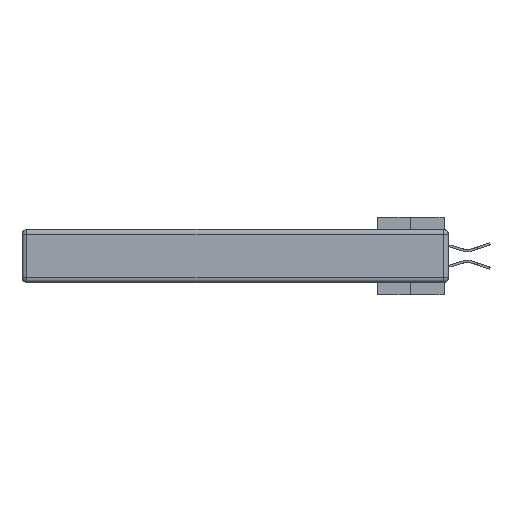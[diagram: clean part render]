
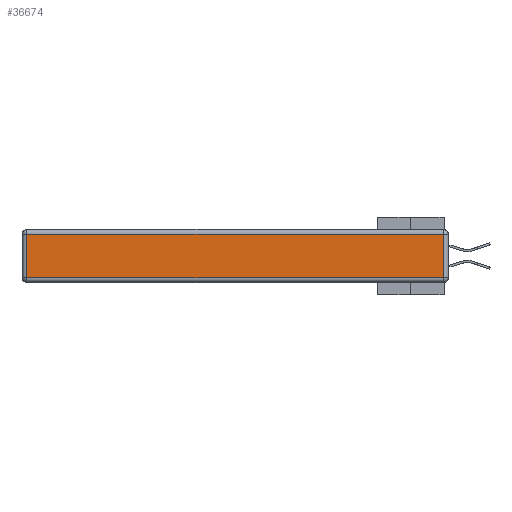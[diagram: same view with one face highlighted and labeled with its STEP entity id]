
A CAD part, left-side view. The second image highlights one B-rep face of the part: STEP entity #36674.
In plain terms, the highlighted planar face has unit normal (-1, 0, 0).
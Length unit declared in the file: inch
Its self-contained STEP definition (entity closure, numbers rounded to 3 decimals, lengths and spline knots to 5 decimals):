
#257 = CARTESIAN_POINT ( 'NONE',  ( 0., 2.72, -0.313 ) ) ;
#616 = VECTOR ( 'NONE', #44466, 39.37008 ) ;
#2462 = VERTEX_POINT ( 'NONE', #24523 ) ;
#2489 = DIRECTION ( 'NONE',  ( 0., 0., 1. ) ) ;
#2950 = CARTESIAN_POINT ( 'NONE',  ( 0., 0., -0.343 ) ) ;
#5806 = CARTESIAN_POINT ( 'NONE',  ( 0., 0.03, -0.03 ) ) ;
#5812 = DIRECTION ( 'NONE',  ( 0., 0., -1. ) ) ;
#9549 = DIRECTION ( 'NONE',  ( 0., 0., 1. ) ) ;
#11667 = AXIS2_PLACEMENT_3D ( 'NONE', #2950, #31925, #2489 ) ;
#12974 = CARTESIAN_POINT ( 'NONE',  ( 0., 2.72, -0.343 ) ) ;
#13382 = DIRECTION ( 'NONE',  ( 0., -1., 0. ) ) ;
#13912 = LINE ( 'NONE', #12974, #41670 ) ;
#15947 = CARTESIAN_POINT ( 'NONE',  ( 0., 2.75, -0.03 ) ) ;
#17008 = ORIENTED_EDGE ( 'NONE', *, *, #37620, .T. ) ;
#17960 = EDGE_LOOP ( 'NONE', ( #41388, #26431, #44806, #17008 ) ) ;
#18274 = LINE ( 'NONE', #28059, #43247 ) ;
#24523 = CARTESIAN_POINT ( 'NONE',  ( 0., 2.72, -0.03 ) ) ;
#26431 = ORIENTED_EDGE ( 'NONE', *, *, #26827, .T. ) ;
#26827 = EDGE_CURVE ( 'NONE', #36642, #41509, #18274, .T. ) ;
#28059 = CARTESIAN_POINT ( 'NONE',  ( 0., 0.03, -0.343 ) ) ;
#28369 = EDGE_CURVE ( 'NONE', #30826, #36642, #46108, .T. ) ;
#30826 = VERTEX_POINT ( 'NONE', #257 ) ;
#31925 = DIRECTION ( 'NONE',  ( -1., 0., 0. ) ) ;
#33640 = VECTOR ( 'NONE', #13382, 39.37008 ) ;
#36642 = VERTEX_POINT ( 'NONE', #42365 ) ;
#36674 = ADVANCED_FACE ( 'NONE', ( #46302 ), #46014, .T. ) ;
#37620 = EDGE_CURVE ( 'NONE', #2462, #30826, #13912, .T. ) ;
#41388 = ORIENTED_EDGE ( 'NONE', *, *, #28369, .T. ) ;
#41446 = EDGE_CURVE ( 'NONE', #41509, #2462, #42547, .T. ) ;
#41509 = VERTEX_POINT ( 'NONE', #5806 ) ;
#41670 = VECTOR ( 'NONE', #5812, 39.37008 ) ;
#42341 = CARTESIAN_POINT ( 'NONE',  ( 0., 0., -0.313 ) ) ;
#42365 = CARTESIAN_POINT ( 'NONE',  ( 0., 0.03, -0.313 ) ) ;
#42547 = LINE ( 'NONE', #15947, #616 ) ;
#43247 = VECTOR ( 'NONE', #9549, 39.37008 ) ;
#44466 = DIRECTION ( 'NONE',  ( 0., 1., 0. ) ) ;
#44806 = ORIENTED_EDGE ( 'NONE', *, *, #41446, .T. ) ;
#46014 = PLANE ( 'NONE',  #11667 ) ;
#46108 = LINE ( 'NONE', #42341, #33640 ) ;
#46302 = FACE_OUTER_BOUND ( 'NONE', #17960, .T. ) ;
